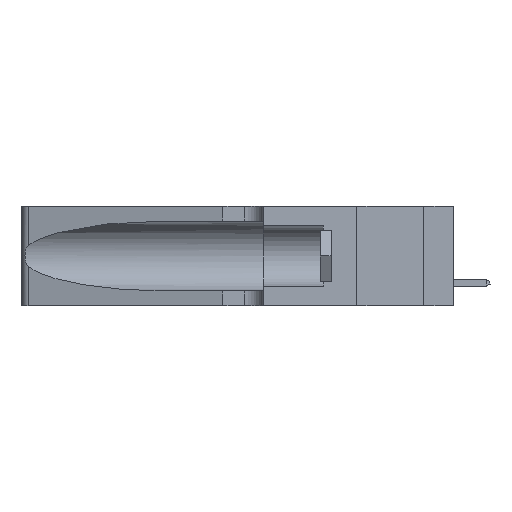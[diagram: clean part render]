
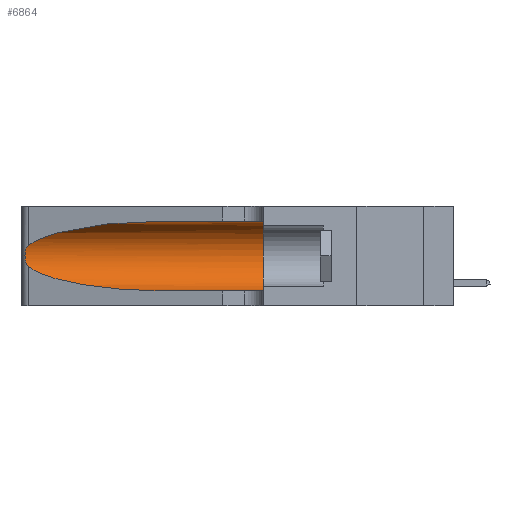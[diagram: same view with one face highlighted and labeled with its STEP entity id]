
A CAD part, left-side view. The second image highlights one B-rep face of the part: STEP entity #6864.
In plain terms, the highlighted cylindrical face has radius 3.308 mm (diameter 6.617 mm), a partial arc.
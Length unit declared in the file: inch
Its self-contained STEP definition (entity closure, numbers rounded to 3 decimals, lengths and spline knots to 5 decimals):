
#146 = CARTESIAN_POINT ( 'NONE',  ( 0.26075, 1.23896, 0.178 ) ) ;
#745 =( BOUNDED_CURVE ( )  B_SPLINE_CURVE ( 3, ( #17911, #37331, #24947, #31234 ),
 .UNSPECIFIED., .F., .F. ) 
 B_SPLINE_CURVE_WITH_KNOTS ( ( 4, 4 ),
 ( 3.44316, 4.71239 ),
 .UNSPECIFIED. ) 
 CURVE ( )  GEOMETRIC_REPRESENTATION_ITEM ( )  RATIONAL_B_SPLINE_CURVE ( ( 1., 0.87, 0.87, 1. ) ) 
 REPRESENTATION_ITEM ( '' )  );
#847 = EDGE_CURVE ( 'NONE', #15700, #19018, #12590, .T. ) ;
#1637 = DIRECTION ( 'NONE',  ( 0., -1., 0. ) ) ;
#2079 = EDGE_CURVE ( 'NONE', #19018, #23714, #24763, .T. ) ;
#2645 = CARTESIAN_POINT ( 'NONE',  ( 0.25787, 1.23484, 0.2124 ) ) ;
#3440 = CARTESIAN_POINT ( 'NONE',  ( 0.26018, 1.23835, 0.19895 ) ) ;
#3593 = CARTESIAN_POINT ( 'NONE',  ( 0.25487, 1.22718, 0.22369 ) ) ;
#4649 = EDGE_CURVE ( 'NONE', #28276, #22300, #7866, .T. ) ;
#5290 = CARTESIAN_POINT ( 'NONE',  ( 0.1305, 0.72297, 0.31525 ) ) ;
#5685 = AXIS2_PLACEMENT_3D ( 'NONE', #34585, #27890, #18756 ) ;
#5736 = FACE_OUTER_BOUND ( 'NONE', #32056, .T. ) ;
#6864 = ADVANCED_FACE ( 'NONE', ( #5736 ), #19887, .F. ) ;
#7659 = EDGE_CURVE ( 'NONE', #23714, #16306, #745, .T. ) ;
#7866 = CIRCLE ( 'NONE', #5685, 0.13025 ) ;
#8146 = CARTESIAN_POINT ( 'NONE',  ( 0.2373, 1.15595, 0.28018 ) ) ;
#8438 = CARTESIAN_POINT ( 'NONE',  ( 0.18966, 0.96281, 0.31525 ) ) ;
#8550 = CARTESIAN_POINT ( 'NONE',  ( 0.1305, 1.61858, 0.31525 ) ) ;
#9045 = DIRECTION ( 'NONE',  ( 0., -1., 0. ) ) ;
#9416 = VECTOR ( 'NONE', #9045, 39.37008 ) ;
#9458 = EDGE_CURVE ( 'NONE', #16306, #22300, #33988, .T. ) ;
#9733 = CARTESIAN_POINT ( 'NONE',  ( 0.25854, 1.2359, 0.20912 ) ) ;
#11477 = AXIS2_PLACEMENT_3D ( 'NONE', #17240, #1637, #21281 ) ;
#12590 =( BOUNDED_CURVE ( )  B_SPLINE_CURVE ( 3, ( #5290, #8438, #8146, #30413 ),
 .UNSPECIFIED., .F., .F. ) 
 B_SPLINE_CURVE_WITH_KNOTS ( ( 4, 4 ),
 ( 1.5708, 2.84003 ),
 .UNSPECIFIED. ) 
 CURVE ( )  GEOMETRIC_REPRESENTATION_ITEM ( )  RATIONAL_B_SPLINE_CURVE ( ( 1., 0.87, 0.87, 1. ) ) 
 REPRESENTATION_ITEM ( '' )  );
#15700 = VERTEX_POINT ( 'NONE', #27738 ) ;
#16108 = ORIENTED_EDGE ( 'NONE', *, *, #30673, .F. ) ;
#16306 = VERTEX_POINT ( 'NONE', #39260 ) ;
#17240 = CARTESIAN_POINT ( 'NONE',  ( 0.1305, 1.61858, 0.185 ) ) ;
#17911 = CARTESIAN_POINT ( 'NONE',  ( 0.25487, 1.22718, 0.14631 ) ) ;
#18259 = CARTESIAN_POINT ( 'NONE',  ( 0.25639, 1.23184, 0.21858 ) ) ;
#18663 = CARTESIAN_POINT ( 'NONE',  ( 0.25789, 1.23486, 0.15765 ) ) ;
#18756 = DIRECTION ( 'NONE',  ( 0., 0., 1. ) ) ;
#19018 = VERTEX_POINT ( 'NONE', #3593 ) ;
#19309 = CARTESIAN_POINT ( 'NONE',  ( 0.25639, 1.23186, 0.15144 ) ) ;
#19887 = CYLINDRICAL_SURFACE ( 'NONE', #11477, 0.13025 ) ;
#21281 = DIRECTION ( 'NONE',  ( 0., 0., -1. ) ) ;
#22182 = LINE ( 'NONE', #8550, #9416 ) ;
#22300 = VERTEX_POINT ( 'NONE', #36547 ) ;
#22634 = CARTESIAN_POINT ( 'NONE',  ( 0.25555, 1.22993, 0.14849 ) ) ;
#22660 = VECTOR ( 'NONE', #35224, 39.37008 ) ;
#23714 = VERTEX_POINT ( 'NONE', #29831 ) ;
#24763 = B_SPLINE_CURVE_WITH_KNOTS ( 'NONE', 3,
 ( #33939, #34355, #18259, #2645, #9733, #3440, #34620, #146, #38075, #28702, #18663, #19309, #22634, #29238 ),
 .UNSPECIFIED., .F., .F.,
 ( 4, 2, 2, 2, 2, 2, 4 ),
 ( 0., 0.00027, 0.00053, 0.00107, 0.0016, 0.00187, 0.00214 ),
 .UNSPECIFIED. ) ;
#24947 = CARTESIAN_POINT ( 'NONE',  ( 0.18966, 0.96281, 0.05475 ) ) ;
#25617 = ORIENTED_EDGE ( 'NONE', *, *, #7659, .T. ) ;
#26755 = ORIENTED_EDGE ( 'NONE', *, *, #4649, .F. ) ;
#27738 = CARTESIAN_POINT ( 'NONE',  ( 0.1305, 0.72297, 0.31525 ) ) ;
#27890 = DIRECTION ( 'NONE',  ( 0., 1., 0. ) ) ;
#28276 = VERTEX_POINT ( 'NONE', #36474 ) ;
#28702 = CARTESIAN_POINT ( 'NONE',  ( 0.25856, 1.23593, 0.16098 ) ) ;
#29238 = CARTESIAN_POINT ( 'NONE',  ( 0.25487, 1.22718, 0.14631 ) ) ;
#29831 = CARTESIAN_POINT ( 'NONE',  ( 0.25487, 1.22718, 0.14631 ) ) ;
#30413 = CARTESIAN_POINT ( 'NONE',  ( 0.25487, 1.22718, 0.22369 ) ) ;
#30514 = ORIENTED_EDGE ( 'NONE', *, *, #2079, .T. ) ;
#30673 = EDGE_CURVE ( 'NONE', #15700, #28276, #22182, .T. ) ;
#31234 = CARTESIAN_POINT ( 'NONE',  ( 0.1305, 0.72297, 0.05475 ) ) ;
#32056 = EDGE_LOOP ( 'NONE', ( #36808, #30514, #25617, #34022, #26755, #16108 ) ) ;
#33939 = CARTESIAN_POINT ( 'NONE',  ( 0.25487, 1.22718, 0.22369 ) ) ;
#33988 = LINE ( 'NONE', #36523, #22660 ) ;
#34022 = ORIENTED_EDGE ( 'NONE', *, *, #9458, .T. ) ;
#34355 = CARTESIAN_POINT ( 'NONE',  ( 0.25555, 1.22994, 0.2215 ) ) ;
#34585 = CARTESIAN_POINT ( 'NONE',  ( 0.1305, 0.35, 0.185 ) ) ;
#34620 = CARTESIAN_POINT ( 'NONE',  ( 0.26075, 1.23896, 0.19203 ) ) ;
#35224 = DIRECTION ( 'NONE',  ( 0., -1., 0. ) ) ;
#36474 = CARTESIAN_POINT ( 'NONE',  ( 0.1305, 0.35, 0.31525 ) ) ;
#36523 = CARTESIAN_POINT ( 'NONE',  ( 0.1305, 1.61858, 0.05475 ) ) ;
#36547 = CARTESIAN_POINT ( 'NONE',  ( 0.1305, 0.35, 0.05475 ) ) ;
#36808 = ORIENTED_EDGE ( 'NONE', *, *, #847, .T. ) ;
#37331 = CARTESIAN_POINT ( 'NONE',  ( 0.2373, 1.15595, 0.08982 ) ) ;
#38075 = CARTESIAN_POINT ( 'NONE',  ( 0.26017, 1.23833, 0.17102 ) ) ;
#39260 = CARTESIAN_POINT ( 'NONE',  ( 0.1305, 0.72297, 0.05475 ) ) ;
